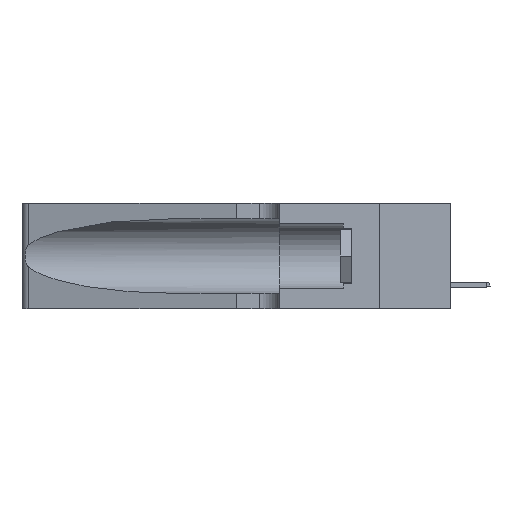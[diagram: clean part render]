
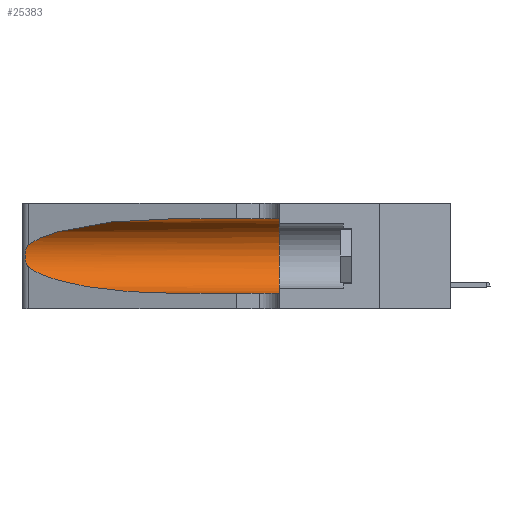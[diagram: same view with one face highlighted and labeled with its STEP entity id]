
A CAD part, left-side view. The second image highlights one B-rep face of the part: STEP entity #25383.
In plain terms, the highlighted cylindrical face has radius 3.308 mm (diameter 6.617 mm), a partial arc.
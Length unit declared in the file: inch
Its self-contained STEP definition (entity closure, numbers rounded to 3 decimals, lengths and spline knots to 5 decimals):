
#44 = CARTESIAN_POINT ( 'NONE',  ( 0.18966, 0.96281, 0.05475 ) ) ;
#376 = VERTEX_POINT ( 'NONE', #25759 ) ;
#495 =( BOUNDED_CURVE ( )  B_SPLINE_CURVE ( 3, ( #21858, #3967, #44, #1878 ),
 .UNSPECIFIED., .F., .T. ) 
 B_SPLINE_CURVE_WITH_KNOTS ( ( 4, 4 ),
 ( 3.44316, 4.71239 ),
 .UNSPECIFIED. ) 
 CURVE ( )  GEOMETRIC_REPRESENTATION_ITEM ( )  RATIONAL_B_SPLINE_CURVE ( ( 1., 0.87, 0.87, 1. ) ) 
 REPRESENTATION_ITEM ( '' )  );
#1012 = ORIENTED_EDGE ( 'NONE', *, *, #19996, .T. ) ;
#1406 = ORIENTED_EDGE ( 'NONE', *, *, #15743, .T. ) ;
#1477 = CARTESIAN_POINT ( 'NONE',  ( 0.26075, 1.23896, 0.178 ) ) ;
#1606 = CARTESIAN_POINT ( 'NONE',  ( 0.26075, 1.23896, 0.19203 ) ) ;
#1878 = CARTESIAN_POINT ( 'NONE',  ( 0.1305, 0.72297, 0.05475 ) ) ;
#2384 = CARTESIAN_POINT ( 'NONE',  ( 0.25555, 1.22993, 0.14849 ) ) ;
#2388 = CARTESIAN_POINT ( 'NONE',  ( 0.1305, 1.61858, 0.185 ) ) ;
#2850 = ORIENTED_EDGE ( 'NONE', *, *, #11229, .F. ) ;
#3002 = VECTOR ( 'NONE', #3994, 39.37008 ) ;
#3233 = AXIS2_PLACEMENT_3D ( 'NONE', #25419, #21891, #15745 ) ;
#3285 = CARTESIAN_POINT ( 'NONE',  ( 0.25487, 1.22718, 0.22369 ) ) ;
#3348 = CARTESIAN_POINT ( 'NONE',  ( 0.1305, 0.72297, 0.31525 ) ) ;
#3490 = VERTEX_POINT ( 'NONE', #20725 ) ;
#3554 = DIRECTION ( 'NONE',  ( 0., -1., 0. ) ) ;
#3967 = CARTESIAN_POINT ( 'NONE',  ( 0.2373, 1.15595, 0.08982 ) ) ;
#3994 = DIRECTION ( 'NONE',  ( 0., -1., 0. ) ) ;
#4571 = CARTESIAN_POINT ( 'NONE',  ( 0.1305, 0.35, 0.31525 ) ) ;
#5693 = CARTESIAN_POINT ( 'NONE',  ( 0.18966, 0.96281, 0.31525 ) ) ;
#6056 = CYLINDRICAL_SURFACE ( 'NONE', #19927, 0.13025 ) ;
#7886 = CARTESIAN_POINT ( 'NONE',  ( 0.26017, 1.23833, 0.17102 ) ) ;
#8145 = FACE_OUTER_BOUND ( 'NONE', #15266, .T. ) ;
#9453 = CARTESIAN_POINT ( 'NONE',  ( 0.25789, 1.23486, 0.15765 ) ) ;
#9580 = CARTESIAN_POINT ( 'NONE',  ( 0.25639, 1.23184, 0.21858 ) ) ;
#9611 = CARTESIAN_POINT ( 'NONE',  ( 0.1305, 1.61858, 0.31525 ) ) ;
#10349 = DIRECTION ( 'NONE',  ( 0., 0., -1. ) ) ;
#11064 = VERTEX_POINT ( 'NONE', #4571 ) ;
#11196 = VERTEX_POINT ( 'NONE', #11695 ) ;
#11229 = EDGE_CURVE ( 'NONE', #376, #11064, #21889, .T. ) ;
#11324 =( BOUNDED_CURVE ( )  B_SPLINE_CURVE ( 3, ( #3348, #5693, #20964, #13129 ),
 .UNSPECIFIED., .F., .F. ) 
 B_SPLINE_CURVE_WITH_KNOTS ( ( 4, 4 ),
 ( 1.5708, 2.84003 ),
 .UNSPECIFIED. ) 
 CURVE ( )  GEOMETRIC_REPRESENTATION_ITEM ( )  RATIONAL_B_SPLINE_CURVE ( ( 1., 0.87, 0.87, 1. ) ) 
 REPRESENTATION_ITEM ( '' )  );
#11486 = VERTEX_POINT ( 'NONE', #12972 ) ;
#11695 = CARTESIAN_POINT ( 'NONE',  ( 0.25487, 1.22718, 0.14631 ) ) ;
#12073 = EDGE_CURVE ( 'NONE', #3490, #11486, #15805, .T. ) ;
#12972 = CARTESIAN_POINT ( 'NONE',  ( 0.1305, 0.35, 0.05475 ) ) ;
#13129 = CARTESIAN_POINT ( 'NONE',  ( 0.25487, 1.22718, 0.22369 ) ) ;
#13745 = CARTESIAN_POINT ( 'NONE',  ( 0.25555, 1.22994, 0.2215 ) ) ;
#13863 = CARTESIAN_POINT ( 'NONE',  ( 0.25856, 1.23593, 0.16098 ) ) ;
#14067 = CIRCLE ( 'NONE', #3233, 0.13025 ) ;
#15266 = EDGE_LOOP ( 'NONE', ( #1406, #25652, #1012, #15954, #16253, #2850 ) ) ;
#15709 = CARTESIAN_POINT ( 'NONE',  ( 0.25487, 1.22718, 0.22369 ) ) ;
#15743 = EDGE_CURVE ( 'NONE', #376, #17957, #11324, .T. ) ;
#15745 = DIRECTION ( 'NONE',  ( 0., 0., 1. ) ) ;
#15805 = LINE ( 'NONE', #17516, #23884 ) ;
#15954 = ORIENTED_EDGE ( 'NONE', *, *, #12073, .T. ) ;
#16253 = ORIENTED_EDGE ( 'NONE', *, *, #24854, .F. ) ;
#17516 = CARTESIAN_POINT ( 'NONE',  ( 0.1305, 1.61858, 0.05475 ) ) ;
#17957 = VERTEX_POINT ( 'NONE', #3285 ) ;
#18729 = EDGE_CURVE ( 'NONE', #17957, #11196, #21017, .T. ) ;
#19361 = CARTESIAN_POINT ( 'NONE',  ( 0.26018, 1.23835, 0.19895 ) ) ;
#19927 = AXIS2_PLACEMENT_3D ( 'NONE', #2388, #21988, #10349 ) ;
#19996 = EDGE_CURVE ( 'NONE', #11196, #3490, #495, .T. ) ;
#20725 = CARTESIAN_POINT ( 'NONE',  ( 0.1305, 0.72297, 0.05475 ) ) ;
#20964 = CARTESIAN_POINT ( 'NONE',  ( 0.2373, 1.15595, 0.28018 ) ) ;
#21017 = B_SPLINE_CURVE_WITH_KNOTS ( 'NONE', 3,
 ( #15709, #13745, #9580, #23811, #25779, #19361, #1606, #1477, #7886, #13863, #9453, #21472, #2384, #21985 ),
 .UNSPECIFIED., .F., .F.,
 ( 4, 2, 2, 2, 2, 2, 4 ),
 ( 0., 0.00027, 0.00053, 0.00107, 0.0016, 0.00187, 0.00214 ),
 .UNSPECIFIED. ) ;
#21472 = CARTESIAN_POINT ( 'NONE',  ( 0.25639, 1.23186, 0.15144 ) ) ;
#21858 = CARTESIAN_POINT ( 'NONE',  ( 0.25487, 1.22718, 0.14631 ) ) ;
#21889 = LINE ( 'NONE', #9611, #3002 ) ;
#21891 = DIRECTION ( 'NONE',  ( 0., 1., 0. ) ) ;
#21985 = CARTESIAN_POINT ( 'NONE',  ( 0.25487, 1.22718, 0.14631 ) ) ;
#21988 = DIRECTION ( 'NONE',  ( 0., -1., 0. ) ) ;
#23811 = CARTESIAN_POINT ( 'NONE',  ( 0.25787, 1.23484, 0.2124 ) ) ;
#23884 = VECTOR ( 'NONE', #3554, 39.37008 ) ;
#24854 = EDGE_CURVE ( 'NONE', #11064, #11486, #14067, .T. ) ;
#25383 = ADVANCED_FACE ( 'NONE', ( #8145 ), #6056, .F. ) ;
#25419 = CARTESIAN_POINT ( 'NONE',  ( 0.1305, 0.35, 0.185 ) ) ;
#25652 = ORIENTED_EDGE ( 'NONE', *, *, #18729, .T. ) ;
#25759 = CARTESIAN_POINT ( 'NONE',  ( 0.1305, 0.72297, 0.31525 ) ) ;
#25779 = CARTESIAN_POINT ( 'NONE',  ( 0.25854, 1.2359, 0.20912 ) ) ;
